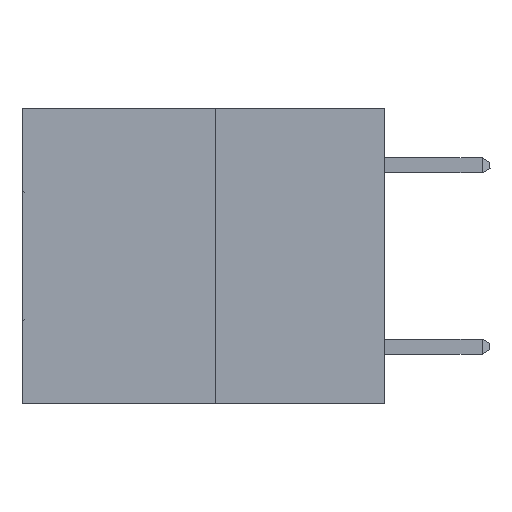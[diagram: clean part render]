
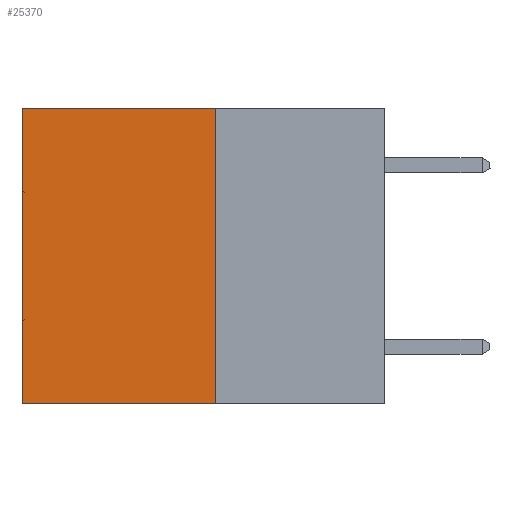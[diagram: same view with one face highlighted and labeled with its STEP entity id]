
A CAD part, left-side view. The second image highlights one B-rep face of the part: STEP entity #25370.
In plain terms, the highlighted planar face has unit normal (-1, 0, 0).
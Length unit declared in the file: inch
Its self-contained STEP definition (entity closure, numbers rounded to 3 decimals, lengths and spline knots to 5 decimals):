
#714 = CARTESIAN_POINT ( 'NONE',  ( 0.3165, 0.6, 0. ) ) ;
#1567 = DIRECTION ( 'NONE',  ( 0., 0., -1. ) ) ;
#2922 = EDGE_CURVE ( 'NONE', #9624, #14688, #24424, .T. ) ;
#3904 = VECTOR ( 'NONE', #23078, 39.37008 ) ;
#3918 = DIRECTION ( 'NONE',  ( 1., 0., 0. ) ) ;
#5922 = DIRECTION ( 'NONE',  ( 0., 0., -1. ) ) ;
#6184 = VERTEX_POINT ( 'NONE', #17576 ) ;
#6624 = FACE_OUTER_BOUND ( 'NONE', #22817, .T. ) ;
#9624 = VERTEX_POINT ( 'NONE', #714 ) ;
#10262 = DIRECTION ( 'NONE',  ( 0., 1., 0. ) ) ;
#11057 = ORIENTED_EDGE ( 'NONE', *, *, #12663, .T. ) ;
#11271 = VERTEX_POINT ( 'NONE', #12013 ) ;
#12013 = CARTESIAN_POINT ( 'NONE',  ( 0.3165, 0.28, 0. ) ) ;
#12137 = DIRECTION ( 'NONE',  ( 0., 0., -1. ) ) ;
#12365 = VECTOR ( 'NONE', #12137, 39.37008 ) ;
#12618 = LINE ( 'NONE', #28124, #3904 ) ;
#12622 = ORIENTED_EDGE ( 'NONE', *, *, #2922, .T. ) ;
#12663 = EDGE_CURVE ( 'NONE', #11271, #9624, #19330, .T. ) ;
#12791 = AXIS2_PLACEMENT_3D ( 'NONE', #24141, #3918, #1567 ) ;
#13528 = LINE ( 'NONE', #27436, #12365 ) ;
#14688 = VERTEX_POINT ( 'NONE', #26330 ) ;
#17576 = CARTESIAN_POINT ( 'NONE',  ( 0.3165, 0.28, -0.49 ) ) ;
#17965 = ORIENTED_EDGE ( 'NONE', *, *, #31850, .F. ) ;
#19086 = PLANE ( 'NONE',  #12791 ) ;
#19330 = LINE ( 'NONE', #30073, #20920 ) ;
#20920 = VECTOR ( 'NONE', #10262, 39.37008 ) ;
#21515 = EDGE_CURVE ( 'NONE', #11271, #6184, #13528, .T. ) ;
#22457 = VECTOR ( 'NONE', #5922, 39.37008 ) ;
#22817 = EDGE_LOOP ( 'NONE', ( #12622, #17965, #27602, #11057 ) ) ;
#23078 = DIRECTION ( 'NONE',  ( 0., 1., 0. ) ) ;
#24141 = CARTESIAN_POINT ( 'NONE',  ( 0.3165, 0.28, -0.49 ) ) ;
#24424 = LINE ( 'NONE', #28519, #22457 ) ;
#25370 = ADVANCED_FACE ( 'NONE', ( #6624 ), #19086, .F. ) ;
#26330 = CARTESIAN_POINT ( 'NONE',  ( 0.3165, 0.6, -0.49 ) ) ;
#27436 = CARTESIAN_POINT ( 'NONE',  ( 0.3165, 0.28, -0.49 ) ) ;
#27602 = ORIENTED_EDGE ( 'NONE', *, *, #21515, .F. ) ;
#28124 = CARTESIAN_POINT ( 'NONE',  ( 0.3165, 0.28, -0.49 ) ) ;
#28519 = CARTESIAN_POINT ( 'NONE',  ( 0.3165, 0.6, -0.49 ) ) ;
#30073 = CARTESIAN_POINT ( 'NONE',  ( 0.3165, 0.28, 0. ) ) ;
#31850 = EDGE_CURVE ( 'NONE', #6184, #14688, #12618, .T. ) ;
